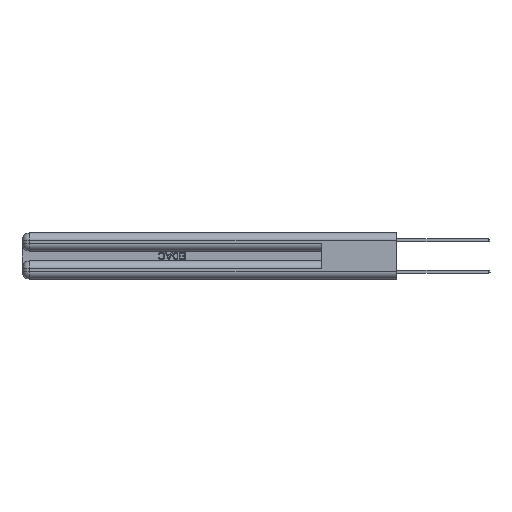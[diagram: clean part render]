
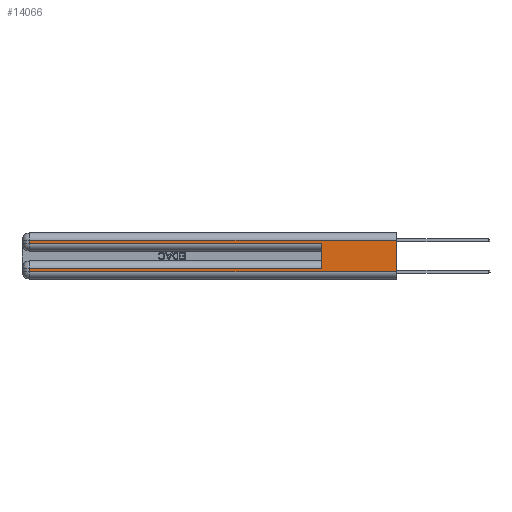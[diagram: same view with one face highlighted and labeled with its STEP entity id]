
A CAD part, left-side view. The second image highlights one B-rep face of the part: STEP entity #14066.
In plain terms, the highlighted planar face has unit normal (-1, 0, 0).
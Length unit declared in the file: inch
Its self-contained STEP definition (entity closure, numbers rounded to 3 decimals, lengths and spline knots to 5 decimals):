
#30 = DIRECTION ( 'NONE',  ( 0., 1., 0. ) ) ;
#961 = DIRECTION ( 'NONE',  ( 0., 1., 0. ) ) ;
#1153 = VERTEX_POINT ( 'NONE', #11411 ) ;
#1685 = CARTESIAN_POINT ( 'NONE',  ( 0., 0., 0.31 ) ) ;
#3771 = DIRECTION ( 'NONE',  ( 0., -1., 0. ) ) ;
#4484 = CARTESIAN_POINT ( 'NONE',  ( 0., 2.94, 0.06 ) ) ;
#5060 = DIRECTION ( 'NONE',  ( 1., 0., 0. ) ) ;
#5099 = CARTESIAN_POINT ( 'NONE',  ( 0., 2.94, 0.37 ) ) ;
#5242 = VECTOR ( 'NONE', #3771, 39.37008 ) ;
#5551 = CARTESIAN_POINT ( 'NONE',  ( 0., 0., 0.31 ) ) ;
#6392 = VERTEX_POINT ( 'NONE', #10937 ) ;
#7213 = EDGE_CURVE ( 'NONE', #23493, #25710, #28635, .T. ) ;
#7505 = CARTESIAN_POINT ( 'NONE',  ( 0., 0., 0.06 ) ) ;
#7809 = LINE ( 'NONE', #20805, #19516 ) ;
#7823 = EDGE_CURVE ( 'NONE', #1153, #20498, #30756, .T. ) ;
#7858 = DIRECTION ( 'NONE',  ( 0., 0., -1. ) ) ;
#7939 = VECTOR ( 'NONE', #34834, 39.37008 ) ;
#7949 = VECTOR ( 'NONE', #30, 39.37008 ) ;
#7997 = EDGE_CURVE ( 'NONE', #1153, #25710, #7809, .T. ) ;
#8141 = VERTEX_POINT ( 'NONE', #1685 ) ;
#8654 = DIRECTION ( 'NONE',  ( 0., 0., -1. ) ) ;
#8941 = ORIENTED_EDGE ( 'NONE', *, *, #25144, .T. ) ;
#9127 = LINE ( 'NONE', #20495, #5242 ) ;
#10937 = CARTESIAN_POINT ( 'NONE',  ( 0., 2.94, 0.31 ) ) ;
#11411 = CARTESIAN_POINT ( 'NONE',  ( 0., 0.6, 0.085 ) ) ;
#11780 = VECTOR ( 'NONE', #25150, 39.37008 ) ;
#11999 = VECTOR ( 'NONE', #8654, 39.37008 ) ;
#13348 = DIRECTION ( 'NONE',  ( 0., 0., -1. ) ) ;
#13453 = VERTEX_POINT ( 'NONE', #4484 ) ;
#13560 = AXIS2_PLACEMENT_3D ( 'NONE', #21640, #5060, #7858 ) ;
#13814 = CARTESIAN_POINT ( 'NONE',  ( 0., 0.6, 0.285 ) ) ;
#14066 = ADVANCED_FACE ( 'NONE', ( #22934 ), #29876, .F. ) ;
#17251 = CARTESIAN_POINT ( 'NONE',  ( 0., 0., 0.085 ) ) ;
#18014 = CARTESIAN_POINT ( 'NONE',  ( 0., 2.94, 0.285 ) ) ;
#18926 = CARTESIAN_POINT ( 'NONE',  ( 0., 2.94, 0.085 ) ) ;
#19198 = LINE ( 'NONE', #26511, #7939 ) ;
#19439 = CARTESIAN_POINT ( 'NONE',  ( 0., 0., 0.285 ) ) ;
#19516 = VECTOR ( 'NONE', #31418, 39.37008 ) ;
#19929 = VECTOR ( 'NONE', #961, 39.37008 ) ;
#20242 = ORIENTED_EDGE ( 'NONE', *, *, #31205, .T. ) ;
#20330 = LINE ( 'NONE', #5099, #34163 ) ;
#20495 = CARTESIAN_POINT ( 'NONE',  ( 0., 0., 0.06 ) ) ;
#20498 = VERTEX_POINT ( 'NONE', #18926 ) ;
#20805 = CARTESIAN_POINT ( 'NONE',  ( 0., 0.6, 0.145 ) ) ;
#20954 = LINE ( 'NONE', #5551, #7949 ) ;
#21640 = CARTESIAN_POINT ( 'NONE',  ( 0., 0., 0.37 ) ) ;
#22322 = CARTESIAN_POINT ( 'NONE',  ( 0., 2.94, 0.37 ) ) ;
#22731 = EDGE_LOOP ( 'NONE', ( #33141, #23523, #8941, #30234, #31149, #29672, #20242, #26882 ) ) ;
#22934 = FACE_OUTER_BOUND ( 'NONE', #22731, .T. ) ;
#23493 = VERTEX_POINT ( 'NONE', #18014 ) ;
#23523 = ORIENTED_EDGE ( 'NONE', *, *, #28649, .T. ) ;
#24372 = VERTEX_POINT ( 'NONE', #7505 ) ;
#25144 = EDGE_CURVE ( 'NONE', #6392, #23493, #20330, .T. ) ;
#25150 = DIRECTION ( 'NONE',  ( 0., -1., 0. ) ) ;
#25710 = VERTEX_POINT ( 'NONE', #13814 ) ;
#26511 = CARTESIAN_POINT ( 'NONE',  ( 0., 0., 0.37 ) ) ;
#26882 = ORIENTED_EDGE ( 'NONE', *, *, #34406, .T. ) ;
#28635 = LINE ( 'NONE', #19439, #11780 ) ;
#28649 = EDGE_CURVE ( 'NONE', #8141, #6392, #20954, .T. ) ;
#29672 = ORIENTED_EDGE ( 'NONE', *, *, #7823, .T. ) ;
#29876 = PLANE ( 'NONE',  #13560 ) ;
#30234 = ORIENTED_EDGE ( 'NONE', *, *, #7213, .T. ) ;
#30756 = LINE ( 'NONE', #17251, #19929 ) ;
#31149 = ORIENTED_EDGE ( 'NONE', *, *, #7997, .F. ) ;
#31205 = EDGE_CURVE ( 'NONE', #20498, #13453, #35324, .T. ) ;
#31418 = DIRECTION ( 'NONE',  ( 0., 0., 1. ) ) ;
#33141 = ORIENTED_EDGE ( 'NONE', *, *, #33462, .F. ) ;
#33462 = EDGE_CURVE ( 'NONE', #8141, #24372, #19198, .T. ) ;
#34163 = VECTOR ( 'NONE', #13348, 39.37008 ) ;
#34406 = EDGE_CURVE ( 'NONE', #13453, #24372, #9127, .T. ) ;
#34834 = DIRECTION ( 'NONE',  ( 0., 0., -1. ) ) ;
#35324 = LINE ( 'NONE', #22322, #11999 ) ;
